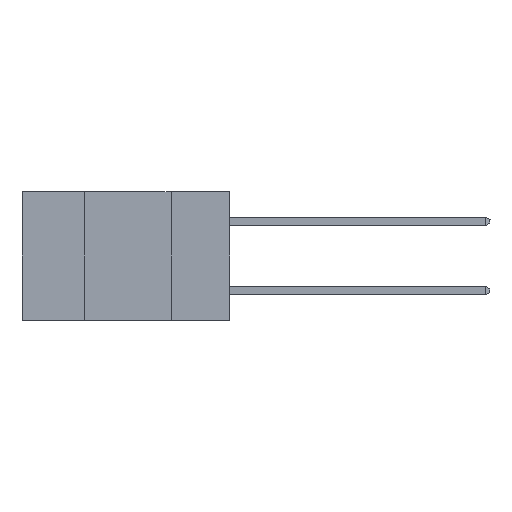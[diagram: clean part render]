
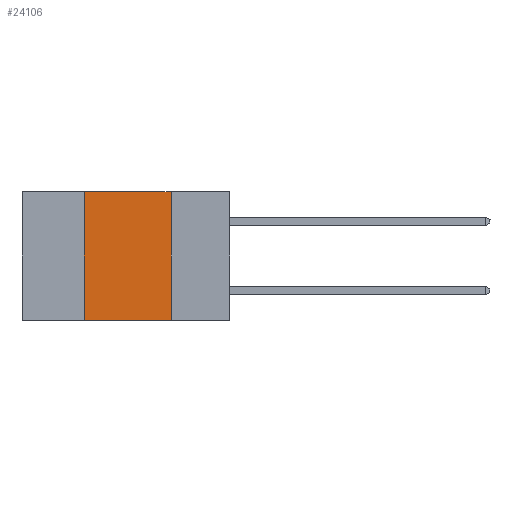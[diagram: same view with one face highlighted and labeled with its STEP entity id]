
A CAD part, left-side view. The second image highlights one B-rep face of the part: STEP entity #24106.
In plain terms, the highlighted planar face has unit normal (-1, 0, 0).
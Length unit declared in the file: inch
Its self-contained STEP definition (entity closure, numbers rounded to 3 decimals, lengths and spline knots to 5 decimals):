
#113 = VERTEX_POINT ( 'NONE', #375 ) ;
#375 = CARTESIAN_POINT ( 'NONE',  ( 0., 0.17, -0.37 ) ) ;
#781 = CARTESIAN_POINT ( 'NONE',  ( 0., 0.42, 0. ) ) ;
#1234 = LINE ( 'NONE', #5483, #10527 ) ;
#1679 = ORIENTED_EDGE ( 'NONE', *, *, #14038, .F. ) ;
#3572 = DIRECTION ( 'NONE',  ( 0., -1., 0. ) ) ;
#4399 = VECTOR ( 'NONE', #12612, 39.37008 ) ;
#4920 = CARTESIAN_POINT ( 'NONE',  ( 0., 0.17, 0. ) ) ;
#5483 = CARTESIAN_POINT ( 'NONE',  ( 0., 0.6, 0. ) ) ;
#5963 = ORIENTED_EDGE ( 'NONE', *, *, #13514, .T. ) ;
#6597 = DIRECTION ( 'NONE',  ( 1., 0., 0. ) ) ;
#6839 = FACE_OUTER_BOUND ( 'NONE', #14542, .T. ) ;
#7666 = ORIENTED_EDGE ( 'NONE', *, *, #7809, .F. ) ;
#7809 = EDGE_CURVE ( 'NONE', #8738, #113, #9379, .T. ) ;
#8738 = VERTEX_POINT ( 'NONE', #15075 ) ;
#9379 = LINE ( 'NONE', #4920, #18977 ) ;
#9551 = CARTESIAN_POINT ( 'NONE',  ( 0., 0.6, -0.37 ) ) ;
#10281 = CARTESIAN_POINT ( 'NONE',  ( 0., 0.42, -0.37 ) ) ;
#10527 = VECTOR ( 'NONE', #3572, 39.37008 ) ;
#11226 = ORIENTED_EDGE ( 'NONE', *, *, #19076, .F. ) ;
#11561 = DIRECTION ( 'NONE',  ( 0., -1., 0. ) ) ;
#12612 = DIRECTION ( 'NONE',  ( 0., 0., 1. ) ) ;
#12980 = VECTOR ( 'NONE', #11561, 39.37008 ) ;
#13514 = EDGE_CURVE ( 'NONE', #16284, #113, #13555, .T. ) ;
#13539 = CARTESIAN_POINT ( 'NONE',  ( 0., 0.42, 0. ) ) ;
#13555 = LINE ( 'NONE', #9551, #12980 ) ;
#14038 = EDGE_CURVE ( 'NONE', #18042, #8738, #1234, .T. ) ;
#14334 = PLANE ( 'NONE',  #22065 ) ;
#14542 = EDGE_LOOP ( 'NONE', ( #7666, #1679, #11226, #5963 ) ) ;
#14774 = LINE ( 'NONE', #781, #4399 ) ;
#15075 = CARTESIAN_POINT ( 'NONE',  ( 0., 0.17, 0. ) ) ;
#16284 = VERTEX_POINT ( 'NONE', #10281 ) ;
#18042 = VERTEX_POINT ( 'NONE', #13539 ) ;
#18135 = DIRECTION ( 'NONE',  ( 0., 0., -1. ) ) ;
#18157 = CARTESIAN_POINT ( 'NONE',  ( 0., 0.6, 0. ) ) ;
#18977 = VECTOR ( 'NONE', #18135, 39.37008 ) ;
#19076 = EDGE_CURVE ( 'NONE', #16284, #18042, #14774, .T. ) ;
#20051 = DIRECTION ( 'NONE',  ( 0., 0., -1. ) ) ;
#22065 = AXIS2_PLACEMENT_3D ( 'NONE', #18157, #6597, #20051 ) ;
#24106 = ADVANCED_FACE ( 'NONE', ( #6839 ), #14334, .F. ) ;
